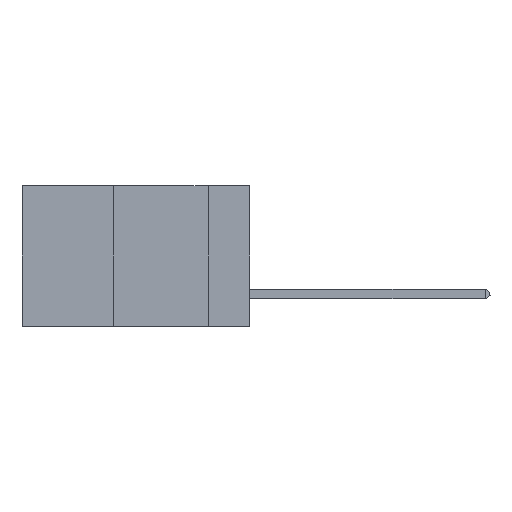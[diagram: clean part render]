
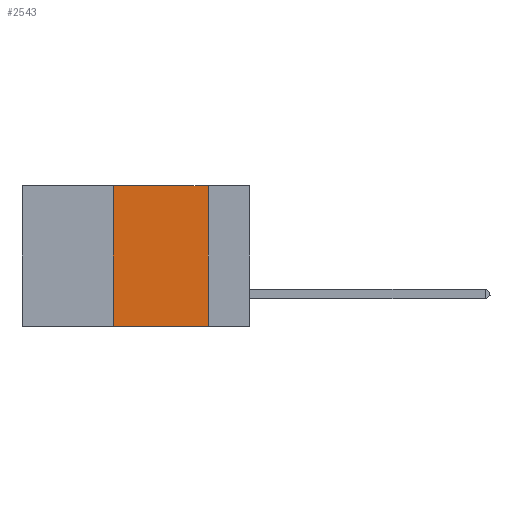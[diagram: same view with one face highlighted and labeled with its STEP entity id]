
A CAD part, left-side view. The second image highlights one B-rep face of the part: STEP entity #2543.
In plain terms, the highlighted planar face has unit normal (-1, 0, 0).
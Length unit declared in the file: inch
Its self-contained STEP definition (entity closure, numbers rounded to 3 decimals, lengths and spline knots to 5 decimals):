
#555 = LINE ( 'NONE', #8905, #20474 ) ;
#1309 = VERTEX_POINT ( 'NONE', #14664 ) ;
#1849 = VECTOR ( 'NONE', #2199, 39.37008 ) ;
#2199 = DIRECTION ( 'NONE',  ( 0., 0., 1. ) ) ;
#2429 = LINE ( 'NONE', #13608, #1849 ) ;
#2543 = ADVANCED_FACE ( 'NONE', ( #9967 ), #10713, .F. ) ;
#3068 = CARTESIAN_POINT ( 'NONE',  ( 0., 0.6, 0. ) ) ;
#3159 = DIRECTION ( 'NONE',  ( 0., 0., -1. ) ) ;
#3681 = VERTEX_POINT ( 'NONE', #23575 ) ;
#4182 = DIRECTION ( 'NONE',  ( 0., -1., 0. ) ) ;
#4258 = ORIENTED_EDGE ( 'NONE', *, *, #17998, .F. ) ;
#4970 = CARTESIAN_POINT ( 'NONE',  ( 0., 0.6, -0.37 ) ) ;
#6205 = ORIENTED_EDGE ( 'NONE', *, *, #19177, .F. ) ;
#6543 = VERTEX_POINT ( 'NONE', #16513 ) ;
#6574 = LINE ( 'NONE', #4970, #7774 ) ;
#7774 = VECTOR ( 'NONE', #8880, 39.37008 ) ;
#8880 = DIRECTION ( 'NONE',  ( 0., -1., 0. ) ) ;
#8905 = CARTESIAN_POINT ( 'NONE',  ( 0., 0.11, 0. ) ) ;
#9106 = VECTOR ( 'NONE', #4182, 39.37008 ) ;
#9659 = EDGE_CURVE ( 'NONE', #6543, #10852, #6574, .T. ) ;
#9967 = FACE_OUTER_BOUND ( 'NONE', #21548, .T. ) ;
#10713 = PLANE ( 'NONE',  #23914 ) ;
#10852 = VERTEX_POINT ( 'NONE', #14290 ) ;
#11886 = CARTESIAN_POINT ( 'NONE',  ( 0., 0.6, 0. ) ) ;
#13605 = ORIENTED_EDGE ( 'NONE', *, *, #24635, .F. ) ;
#13608 = CARTESIAN_POINT ( 'NONE',  ( 0., 0.36, 0. ) ) ;
#14290 = CARTESIAN_POINT ( 'NONE',  ( 0., 0.11, -0.37 ) ) ;
#14664 = CARTESIAN_POINT ( 'NONE',  ( 0., 0.36, 0. ) ) ;
#16513 = CARTESIAN_POINT ( 'NONE',  ( 0., 0.36, -0.37 ) ) ;
#16519 = DIRECTION ( 'NONE',  ( 1., 0., 0. ) ) ;
#17998 = EDGE_CURVE ( 'NONE', #6543, #1309, #2429, .T. ) ;
#18508 = LINE ( 'NONE', #11886, #9106 ) ;
#19177 = EDGE_CURVE ( 'NONE', #1309, #3681, #18508, .T. ) ;
#20474 = VECTOR ( 'NONE', #22346, 39.37008 ) ;
#21548 = EDGE_LOOP ( 'NONE', ( #13605, #6205, #4258, #24775 ) ) ;
#22346 = DIRECTION ( 'NONE',  ( 0., 0., -1. ) ) ;
#23575 = CARTESIAN_POINT ( 'NONE',  ( 0., 0.11, 0. ) ) ;
#23914 = AXIS2_PLACEMENT_3D ( 'NONE', #3068, #16519, #3159 ) ;
#24635 = EDGE_CURVE ( 'NONE', #3681, #10852, #555, .T. ) ;
#24775 = ORIENTED_EDGE ( 'NONE', *, *, #9659, .T. ) ;
